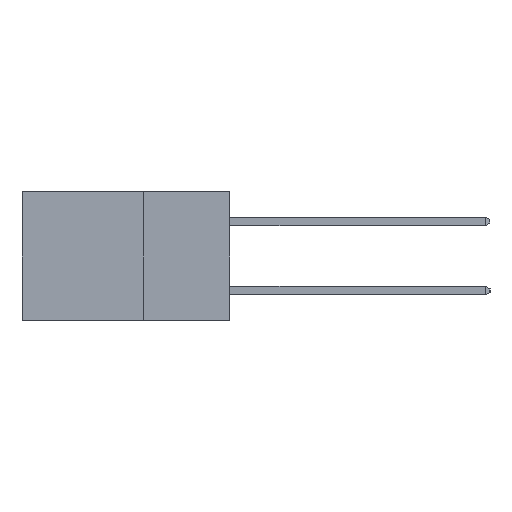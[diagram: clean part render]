
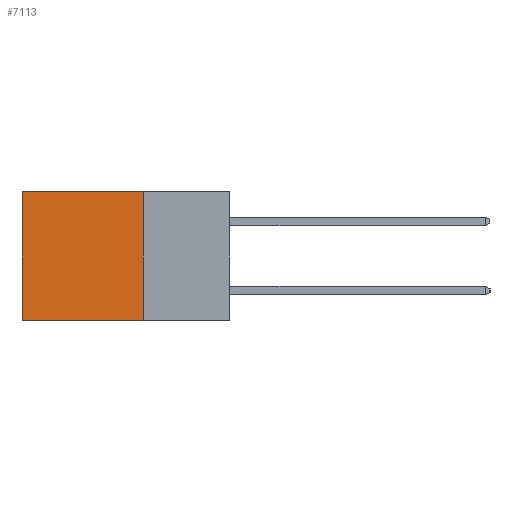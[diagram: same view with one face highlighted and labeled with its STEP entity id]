
A CAD part, left-side view. The second image highlights one B-rep face of the part: STEP entity #7113.
In plain terms, the highlighted planar face has unit normal (-1, 0, 0).
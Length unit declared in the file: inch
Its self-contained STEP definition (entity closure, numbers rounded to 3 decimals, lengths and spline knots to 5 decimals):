
#805 = PLANE ( 'NONE',  #6799 ) ;
#839 = LINE ( 'NONE', #7122, #2298 ) ;
#1151 = CARTESIAN_POINT ( 'NONE',  ( 0.2615, 0.25, 0. ) ) ;
#1668 = LINE ( 'NONE', #2611, #8933 ) ;
#1706 = DIRECTION ( 'NONE',  ( 0., 0., -1. ) ) ;
#1834 = LINE ( 'NONE', #7198, #7906 ) ;
#2298 = VECTOR ( 'NONE', #8003, 39.37008 ) ;
#2375 = EDGE_CURVE ( 'NONE', #4088, #5142, #1834, .T. ) ;
#2574 = ORIENTED_EDGE ( 'NONE', *, *, #2375, .F. ) ;
#2603 = ORIENTED_EDGE ( 'NONE', *, *, #3207, .F. ) ;
#2611 = CARTESIAN_POINT ( 'NONE',  ( 0.2615, 0.25, -0.37 ) ) ;
#3207 = EDGE_CURVE ( 'NONE', #5318, #4088, #1668, .T. ) ;
#3407 = DIRECTION ( 'NONE',  ( 0., 0., -1. ) ) ;
#4088 = VERTEX_POINT ( 'NONE', #6278 ) ;
#5089 = CARTESIAN_POINT ( 'NONE',  ( 0.2615, 0.6, -0.37 ) ) ;
#5142 = VERTEX_POINT ( 'NONE', #10901 ) ;
#5318 = VERTEX_POINT ( 'NONE', #1151 ) ;
#5363 = CARTESIAN_POINT ( 'NONE',  ( 0.2615, 0.6, 0. ) ) ;
#5447 = FACE_OUTER_BOUND ( 'NONE', #9801, .T. ) ;
#5520 = EDGE_CURVE ( 'NONE', #5318, #7992, #839, .T. ) ;
#6278 = CARTESIAN_POINT ( 'NONE',  ( 0.2615, 0.25, -0.37 ) ) ;
#6799 = AXIS2_PLACEMENT_3D ( 'NONE', #9370, #8473, #9410 ) ;
#6940 = VECTOR ( 'NONE', #3407, 39.37008 ) ;
#7014 = EDGE_CURVE ( 'NONE', #7992, #5142, #7201, .T. ) ;
#7113 = ADVANCED_FACE ( 'NONE', ( #5447 ), #805, .F. ) ;
#7122 = CARTESIAN_POINT ( 'NONE',  ( 0.2615, 0.25, 0. ) ) ;
#7198 = CARTESIAN_POINT ( 'NONE',  ( 0.2615, 0.25, -0.37 ) ) ;
#7201 = LINE ( 'NONE', #5089, #6940 ) ;
#7906 = VECTOR ( 'NONE', #9812, 39.37008 ) ;
#7992 = VERTEX_POINT ( 'NONE', #5363 ) ;
#8003 = DIRECTION ( 'NONE',  ( 0., 1., 0. ) ) ;
#8114 = ORIENTED_EDGE ( 'NONE', *, *, #5520, .T. ) ;
#8473 = DIRECTION ( 'NONE',  ( 1., 0., 0. ) ) ;
#8933 = VECTOR ( 'NONE', #1706, 39.37008 ) ;
#9370 = CARTESIAN_POINT ( 'NONE',  ( 0.2615, 0.25, -0.37 ) ) ;
#9410 = DIRECTION ( 'NONE',  ( 0., 0., -1. ) ) ;
#9801 = EDGE_LOOP ( 'NONE', ( #10410, #2574, #2603, #8114 ) ) ;
#9812 = DIRECTION ( 'NONE',  ( 0., 1., 0. ) ) ;
#10410 = ORIENTED_EDGE ( 'NONE', *, *, #7014, .T. ) ;
#10901 = CARTESIAN_POINT ( 'NONE',  ( 0.2615, 0.6, -0.37 ) ) ;
